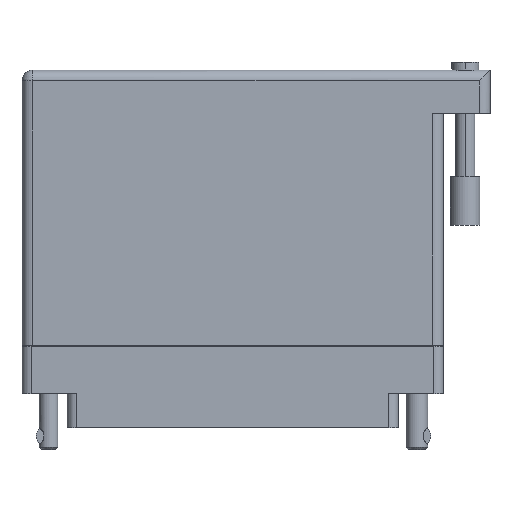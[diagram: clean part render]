
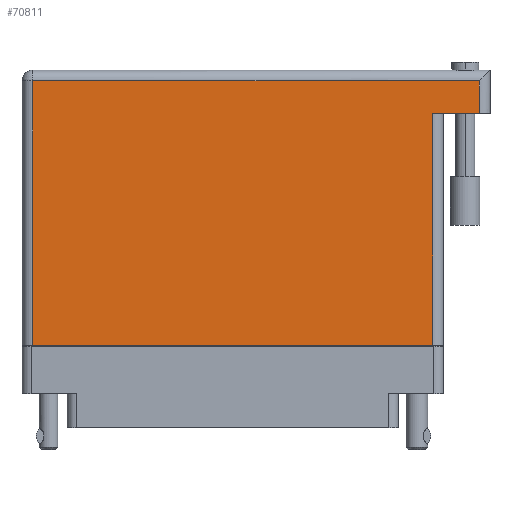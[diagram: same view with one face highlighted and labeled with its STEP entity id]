
A CAD part, front view. The second image highlights one B-rep face of the part: STEP entity #70811.
In plain terms, the highlighted face is planar.
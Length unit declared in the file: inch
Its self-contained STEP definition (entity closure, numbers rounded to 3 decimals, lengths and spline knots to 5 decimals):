
#2 = DIRECTION ( 'NONE',  ( 0., 0., -1. ) ) ;
#263 = PLANE ( 'NONE',  #14957 ) ;
#1409 = VECTOR ( 'NONE', #9474, 39.37008 ) ;
#5131 = LINE ( 'NONE', #28063, #1409 ) ;
#8771 = ORIENTED_EDGE ( 'NONE', *, *, #25263, .T. ) ;
#9474 = DIRECTION ( 'NONE',  ( 0., -1., 0. ) ) ;
#10527 = LINE ( 'NONE', #55762, #51178 ) ;
#14433 = CARTESIAN_POINT ( 'NONE',  ( 1.289, -0.1, 0.617 ) ) ;
#14596 = VECTOR ( 'NONE', #46338, 39.37008 ) ;
#14957 = AXIS2_PLACEMENT_3D ( 'NONE', #36213, #2, #54101 ) ;
#15455 = EDGE_CURVE ( 'NONE', #25375, #35441, #10527, .T. ) ;
#17937 = CARTESIAN_POINT ( 'NONE',  ( 1.589, 1.395, 0.617 ) ) ;
#18983 = ORIENTED_EDGE ( 'NONE', *, *, #25547, .F. ) ;
#25263 = EDGE_CURVE ( 'NONE', #43700, #48514, #71560, .T. ) ;
#25357 = VECTOR ( 'NONE', #58718, 39.37008 ) ;
#25375 = VERTEX_POINT ( 'NONE', #14433 ) ;
#25547 = EDGE_CURVE ( 'NONE', #70847, #35441, #66791, .T. ) ;
#25998 = CARTESIAN_POINT ( 'NONE',  ( -1.359, -0.1, 0.617 ) ) ;
#27409 = EDGE_CURVE ( 'NONE', #70847, #43700, #55171, .T. ) ;
#28063 = CARTESIAN_POINT ( 'NONE',  ( -1.289, -0.1, 0.617 ) ) ;
#29197 = VECTOR ( 'NONE', #49571, 39.37008 ) ;
#32074 = DIRECTION ( 'NONE',  ( 0., 1., 0. ) ) ;
#35441 = VERTEX_POINT ( 'NONE', #52632 ) ;
#35728 = EDGE_CURVE ( 'NONE', #55370, #25375, #65446, .T. ) ;
#36213 = CARTESIAN_POINT ( 'NONE',  ( -1.359, 1.675, 0.617 ) ) ;
#43522 = ORIENTED_EDGE ( 'NONE', *, *, #35728, .T. ) ;
#43700 = VERTEX_POINT ( 'NONE', #56565 ) ;
#44220 = FACE_OUTER_BOUND ( 'NONE', #68689, .T. ) ;
#46338 = DIRECTION ( 'NONE',  ( 0., 1., 0. ) ) ;
#47395 = CARTESIAN_POINT ( 'NONE',  ( 1.659, 1.395, 0.617 ) ) ;
#48514 = VERTEX_POINT ( 'NONE', #76380 ) ;
#49571 = DIRECTION ( 'NONE',  ( -1., 0., 0. ) ) ;
#51178 = VECTOR ( 'NONE', #32074, 39.37008 ) ;
#52632 = CARTESIAN_POINT ( 'NONE',  ( 1.289, 1.395, 0.617 ) ) ;
#54101 = DIRECTION ( 'NONE',  ( -1., 0., 0. ) ) ;
#55171 = LINE ( 'NONE', #77669, #14596 ) ;
#55279 = ORIENTED_EDGE ( 'NONE', *, *, #15455, .T. ) ;
#55370 = VERTEX_POINT ( 'NONE', #73635 ) ;
#55762 = CARTESIAN_POINT ( 'NONE',  ( 1.289, 1.395, 0.617 ) ) ;
#56565 = CARTESIAN_POINT ( 'NONE',  ( 1.589, 1.605, 0.617 ) ) ;
#56982 = VECTOR ( 'NONE', #67563, 39.37008 ) ;
#58718 = DIRECTION ( 'NONE',  ( -1., 0., 0. ) ) ;
#61699 = ORIENTED_EDGE ( 'NONE', *, *, #27409, .T. ) ;
#62455 = CARTESIAN_POINT ( 'NONE',  ( -1.359, 1.605, 0.617 ) ) ;
#65446 = LINE ( 'NONE', #25998, #56982 ) ;
#66570 = EDGE_CURVE ( 'NONE', #48514, #55370, #5131, .T. ) ;
#66791 = LINE ( 'NONE', #47395, #25357 ) ;
#67563 = DIRECTION ( 'NONE',  ( 1., 0., 0. ) ) ;
#68689 = EDGE_LOOP ( 'NONE', ( #43522, #55279, #18983, #61699, #8771, #75847 ) ) ;
#70811 = ADVANCED_FACE ( 'NONE', ( #44220 ), #263, .F. ) ;
#70847 = VERTEX_POINT ( 'NONE', #17937 ) ;
#71560 = LINE ( 'NONE', #62455, #29197 ) ;
#73635 = CARTESIAN_POINT ( 'NONE',  ( -1.289, -0.1, 0.617 ) ) ;
#75847 = ORIENTED_EDGE ( 'NONE', *, *, #66570, .T. ) ;
#76380 = CARTESIAN_POINT ( 'NONE',  ( -1.289, 1.605, 0.617 ) ) ;
#77669 = CARTESIAN_POINT ( 'NONE',  ( 1.589, 1.675, 0.617 ) ) ;
